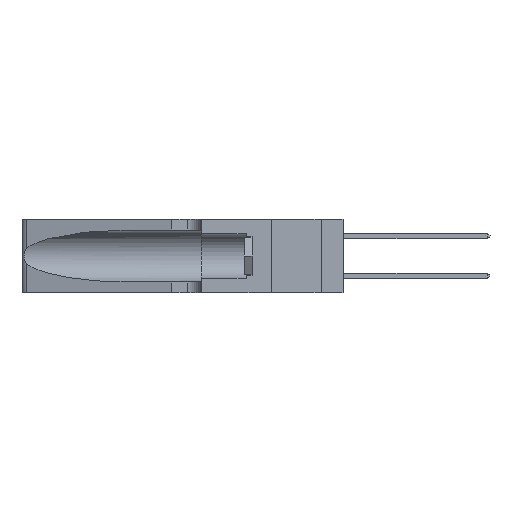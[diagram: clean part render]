
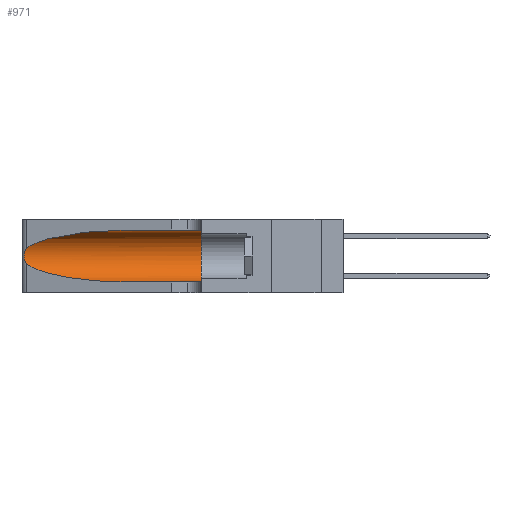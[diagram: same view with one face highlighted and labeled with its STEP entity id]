
A CAD part, left-side view. The second image highlights one B-rep face of the part: STEP entity #971.
In plain terms, the highlighted cylindrical face has radius 3.308 mm (diameter 6.617 mm), a partial arc.
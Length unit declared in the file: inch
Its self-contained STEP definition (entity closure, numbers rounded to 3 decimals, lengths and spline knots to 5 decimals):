
#194 = VERTEX_POINT ( 'NONE', #16810 ) ;
#270 = CARTESIAN_POINT ( 'NONE',  ( 0.18966, 0.96281, 0.31525 ) ) ;
#584 = ORIENTED_EDGE ( 'NONE', *, *, #10730, .T. ) ;
#971 = ADVANCED_FACE ( 'NONE', ( #2796 ), #24353, .F. ) ;
#1028 = CARTESIAN_POINT ( 'NONE',  ( 0.1305, 1.61858, 0.185 ) ) ;
#1724 = AXIS2_PLACEMENT_3D ( 'NONE', #1028, #21396, #14512 ) ;
#2327 = VERTEX_POINT ( 'NONE', #17877 ) ;
#2517 = ORIENTED_EDGE ( 'NONE', *, *, #8439, .F. ) ;
#2578 = EDGE_CURVE ( 'NONE', #194, #2327, #17976, .T. ) ;
#2657 = VERTEX_POINT ( 'NONE', #23384 ) ;
#2796 = FACE_OUTER_BOUND ( 'NONE', #16030, .T. ) ;
#4063 = CARTESIAN_POINT ( 'NONE',  ( 0.25487, 1.22718, 0.22369 ) ) ;
#4182 = EDGE_CURVE ( 'NONE', #28721, #2657, #7886, .T. ) ;
#4261 = CARTESIAN_POINT ( 'NONE',  ( 0.1305, 1.61858, 0.05475 ) ) ;
#5690 = ORIENTED_EDGE ( 'NONE', *, *, #2578, .T. ) ;
#6341 = CARTESIAN_POINT ( 'NONE',  ( 0.25854, 1.2359, 0.20912 ) ) ;
#6536 = CARTESIAN_POINT ( 'NONE',  ( 0.26017, 1.23833, 0.17102 ) ) ;
#7886 =( BOUNDED_CURVE ( )  B_SPLINE_CURVE ( 3, ( #9463, #270, #11706, #27530 ),
 .UNSPECIFIED., .F., .F. ) 
 B_SPLINE_CURVE_WITH_KNOTS ( ( 4, 4 ),
 ( 1.5708, 2.84003 ),
 .UNSPECIFIED. ) 
 CURVE ( )  GEOMETRIC_REPRESENTATION_ITEM ( )  RATIONAL_B_SPLINE_CURVE ( ( 1., 0.87, 0.87, 1. ) ) 
 REPRESENTATION_ITEM ( '' )  );
#8439 = EDGE_CURVE ( 'NONE', #28721, #13456, #23390, .T. ) ;
#8780 = CARTESIAN_POINT ( 'NONE',  ( 0.25856, 1.23593, 0.16098 ) ) ;
#8888 = DIRECTION ( 'NONE',  ( 0., -1., 0. ) ) ;
#8894 = ORIENTED_EDGE ( 'NONE', *, *, #15280, .T. ) ;
#9142 = VECTOR ( 'NONE', #8888, 39.37008 ) ;
#9463 = CARTESIAN_POINT ( 'NONE',  ( 0.1305, 0.72297, 0.31525 ) ) ;
#10730 = EDGE_CURVE ( 'NONE', #2327, #20770, #21072, .T. ) ;
#10925 = CARTESIAN_POINT ( 'NONE',  ( 0.1305, 0.35, 0.31525 ) ) ;
#11706 = CARTESIAN_POINT ( 'NONE',  ( 0.2373, 1.15595, 0.28018 ) ) ;
#11955 = CARTESIAN_POINT ( 'NONE',  ( 0.1305, 0.35, 0.185 ) ) ;
#12147 = CARTESIAN_POINT ( 'NONE',  ( 0.1305, 1.61858, 0.31525 ) ) ;
#12265 = CARTESIAN_POINT ( 'NONE',  ( 0.18966, 0.96281, 0.05475 ) ) ;
#13207 = CARTESIAN_POINT ( 'NONE',  ( 0.25639, 1.23186, 0.15144 ) ) ;
#13456 = VERTEX_POINT ( 'NONE', #10925 ) ;
#14217 = DIRECTION ( 'NONE',  ( 0., 0., 1. ) ) ;
#14512 = DIRECTION ( 'NONE',  ( 0., 0., -1. ) ) ;
#14680 = CARTESIAN_POINT ( 'NONE',  ( 0.1305, 0.72297, 0.31525 ) ) ;
#14809 = CARTESIAN_POINT ( 'NONE',  ( 0.25487, 1.22718, 0.14631 ) ) ;
#14904 = EDGE_CURVE ( 'NONE', #13456, #20770, #23816, .T. ) ;
#15006 = CARTESIAN_POINT ( 'NONE',  ( 0.1305, 0.35, 0.05475 ) ) ;
#15280 = EDGE_CURVE ( 'NONE', #2657, #194, #17070, .T. ) ;
#16030 = EDGE_LOOP ( 'NONE', ( #24433, #8894, #5690, #584, #21696, #2517 ) ) ;
#16810 = CARTESIAN_POINT ( 'NONE',  ( 0.25487, 1.22718, 0.14631 ) ) ;
#16967 = CARTESIAN_POINT ( 'NONE',  ( 0.2373, 1.15595, 0.08982 ) ) ;
#17063 = CARTESIAN_POINT ( 'NONE',  ( 0.1305, 0.72297, 0.05475 ) ) ;
#17070 = B_SPLINE_CURVE_WITH_KNOTS ( 'NONE', 3,
 ( #4063, #22172, #28916, #26759, #6341, #26548, #19968, #17821, #6536, #8780, #24585, #13207, #20075, #26953 ),
 .UNSPECIFIED., .F., .F.,
 ( 4, 2, 2, 2, 2, 2, 4 ),
 ( 0., 0.00027, 0.00053, 0.00107, 0.0016, 0.00187, 0.00214 ),
 .UNSPECIFIED. ) ;
#17821 = CARTESIAN_POINT ( 'NONE',  ( 0.26075, 1.23896, 0.178 ) ) ;
#17877 = CARTESIAN_POINT ( 'NONE',  ( 0.1305, 0.72297, 0.05475 ) ) ;
#17976 =( BOUNDED_CURVE ( )  B_SPLINE_CURVE ( 3, ( #14809, #16967, #12265, #17063 ),
 .UNSPECIFIED., .F., .F. ) 
 B_SPLINE_CURVE_WITH_KNOTS ( ( 4, 4 ),
 ( 3.44316, 4.71239 ),
 .UNSPECIFIED. ) 
 CURVE ( )  GEOMETRIC_REPRESENTATION_ITEM ( )  RATIONAL_B_SPLINE_CURVE ( ( 1., 0.87, 0.87, 1. ) ) 
 REPRESENTATION_ITEM ( '' )  );
#19968 = CARTESIAN_POINT ( 'NONE',  ( 0.26075, 1.23896, 0.19203 ) ) ;
#20075 = CARTESIAN_POINT ( 'NONE',  ( 0.25555, 1.22993, 0.14849 ) ) ;
#20770 = VERTEX_POINT ( 'NONE', #15006 ) ;
#21072 = LINE ( 'NONE', #4261, #9142 ) ;
#21396 = DIRECTION ( 'NONE',  ( 0., -1., 0. ) ) ;
#21696 = ORIENTED_EDGE ( 'NONE', *, *, #14904, .F. ) ;
#22172 = CARTESIAN_POINT ( 'NONE',  ( 0.25555, 1.22994, 0.2215 ) ) ;
#22650 = VECTOR ( 'NONE', #27677, 39.37008 ) ;
#23384 = CARTESIAN_POINT ( 'NONE',  ( 0.25487, 1.22718, 0.22369 ) ) ;
#23390 = LINE ( 'NONE', #12147, #22650 ) ;
#23816 = CIRCLE ( 'NONE', #26026, 0.13025 ) ;
#24353 = CYLINDRICAL_SURFACE ( 'NONE', #1724, 0.13025 ) ;
#24433 = ORIENTED_EDGE ( 'NONE', *, *, #4182, .T. ) ;
#24585 = CARTESIAN_POINT ( 'NONE',  ( 0.25789, 1.23486, 0.15765 ) ) ;
#25215 = DIRECTION ( 'NONE',  ( 0., 1., 0. ) ) ;
#26026 = AXIS2_PLACEMENT_3D ( 'NONE', #11955, #25215, #14217 ) ;
#26548 = CARTESIAN_POINT ( 'NONE',  ( 0.26018, 1.23835, 0.19895 ) ) ;
#26759 = CARTESIAN_POINT ( 'NONE',  ( 0.25787, 1.23484, 0.2124 ) ) ;
#26953 = CARTESIAN_POINT ( 'NONE',  ( 0.25487, 1.22718, 0.14631 ) ) ;
#27530 = CARTESIAN_POINT ( 'NONE',  ( 0.25487, 1.22718, 0.22369 ) ) ;
#27677 = DIRECTION ( 'NONE',  ( 0., -1., 0. ) ) ;
#28721 = VERTEX_POINT ( 'NONE', #14680 ) ;
#28916 = CARTESIAN_POINT ( 'NONE',  ( 0.25639, 1.23184, 0.21858 ) ) ;
